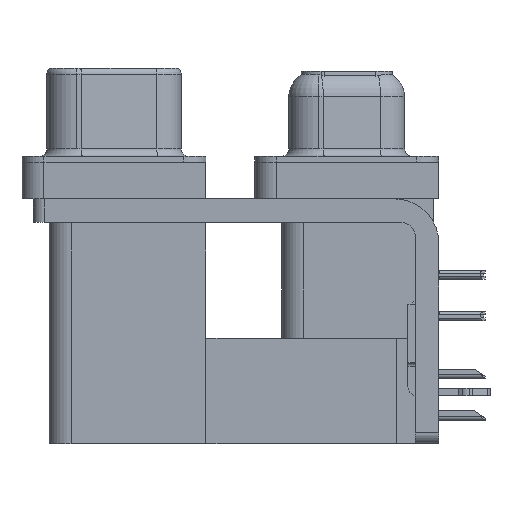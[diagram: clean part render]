
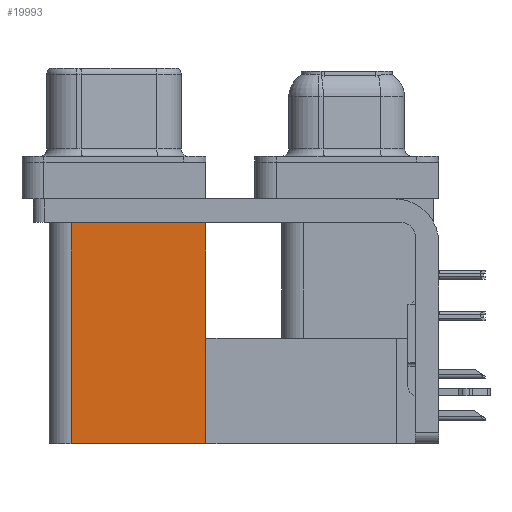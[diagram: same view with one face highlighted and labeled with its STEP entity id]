
A CAD part, left-side view. The second image highlights one B-rep face of the part: STEP entity #19993.
In plain terms, the highlighted planar face has unit normal (-1, 0, 0).
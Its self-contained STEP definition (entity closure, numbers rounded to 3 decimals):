
#1092 = DIRECTION ( 'NONE',  ( 0., 0., -1. ) ) ;
#2570 = EDGE_CURVE ( 'NONE', #20740, #44190, #38195, .T. ) ;
#4104 = EDGE_CURVE ( 'NONE', #20740, #30190, #22990, .T. ) ;
#5533 = CARTESIAN_POINT ( 'NONE',  ( 3.765, 9.6, -2.5 ) ) ;
#6038 = CARTESIAN_POINT ( 'NONE',  ( 3.765, 9.6, -19.2 ) ) ;
#6392 = CARTESIAN_POINT ( 'NONE',  ( 3.765, 9.6, -19.2 ) ) ;
#6394 = ORIENTED_EDGE ( 'NONE', *, *, #42452, .T. ) ;
#7089 = LINE ( 'NONE', #25427, #29798 ) ;
#8724 = CARTESIAN_POINT ( 'NONE',  ( 3.765, 9.6, -2.5 ) ) ;
#10122 = ORIENTED_EDGE ( 'NONE', *, *, #2570, .T. ) ;
#11488 = DIRECTION ( 'NONE',  ( 0., 0., 1. ) ) ;
#14813 = PLANE ( 'NONE',  #39142 ) ;
#16274 = VECTOR ( 'NONE', #27749, 1000. ) ;
#19993 = ADVANCED_FACE ( 'NONE', ( #35921 ), #14813, .F. ) ;
#20740 = VERTEX_POINT ( 'NONE', #32939 ) ;
#22990 = LINE ( 'NONE', #6038, #42373 ) ;
#24442 = EDGE_CURVE ( 'NONE', #30190, #35810, #7089, .T. ) ;
#25427 = CARTESIAN_POINT ( 'NONE',  ( 3.765, 18.8, -19.2 ) ) ;
#27749 = DIRECTION ( 'NONE',  ( 0., 0., 1. ) ) ;
#28946 = CARTESIAN_POINT ( 'NONE',  ( 3.765, 9.6, -19.2 ) ) ;
#29798 = VECTOR ( 'NONE', #11488, 1000. ) ;
#30059 = DIRECTION ( 'NONE',  ( 0., 1., 0. ) ) ;
#30190 = VERTEX_POINT ( 'NONE', #38218 ) ;
#32939 = CARTESIAN_POINT ( 'NONE',  ( 3.765, 9.6, -19.2 ) ) ;
#34115 = DIRECTION ( 'NONE',  ( 0., 1., 0. ) ) ;
#35369 = VECTOR ( 'NONE', #30059, 1000. ) ;
#35459 = LINE ( 'NONE', #8724, #35369 ) ;
#35810 = VERTEX_POINT ( 'NONE', #43083 ) ;
#35921 = FACE_OUTER_BOUND ( 'NONE', #39859, .T. ) ;
#38195 = LINE ( 'NONE', #6392, #16274 ) ;
#38218 = CARTESIAN_POINT ( 'NONE',  ( 3.765, 18.8, -19.2 ) ) ;
#38568 = ORIENTED_EDGE ( 'NONE', *, *, #24442, .F. ) ;
#39142 = AXIS2_PLACEMENT_3D ( 'NONE', #28946, #42884, #1092 ) ;
#39859 = EDGE_LOOP ( 'NONE', ( #6394, #38568, #45850, #10122 ) ) ;
#42373 = VECTOR ( 'NONE', #34115, 1000. ) ;
#42452 = EDGE_CURVE ( 'NONE', #44190, #35810, #35459, .T. ) ;
#42884 = DIRECTION ( 'NONE',  ( 1., 0., 0. ) ) ;
#43083 = CARTESIAN_POINT ( 'NONE',  ( 3.765, 18.8, -2.5 ) ) ;
#44190 = VERTEX_POINT ( 'NONE', #5533 ) ;
#45850 = ORIENTED_EDGE ( 'NONE', *, *, #4104, .F. ) ;
